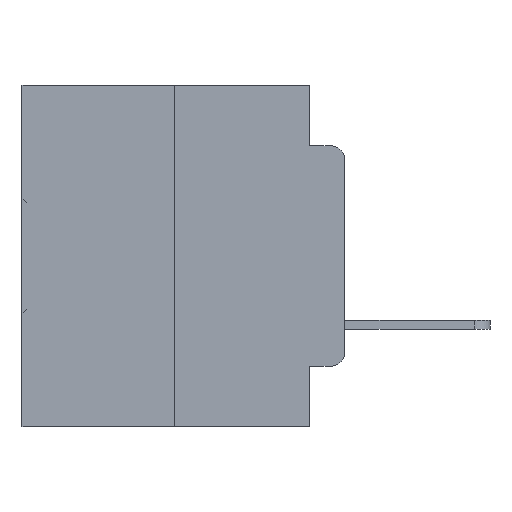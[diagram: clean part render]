
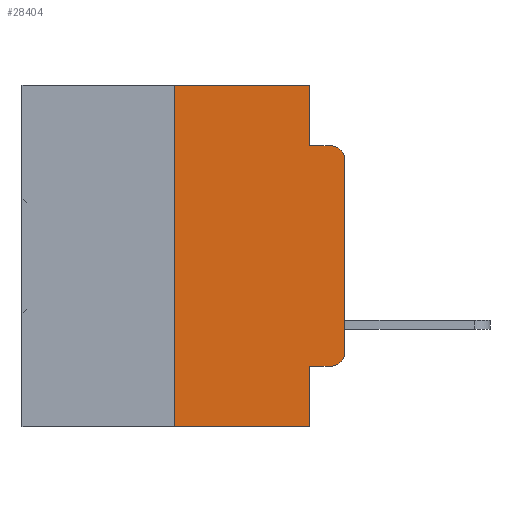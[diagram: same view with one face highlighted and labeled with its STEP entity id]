
A CAD part, left-side view. The second image highlights one B-rep face of the part: STEP entity #28404.
In plain terms, the highlighted planar face has unit normal (-1, 0, 0).
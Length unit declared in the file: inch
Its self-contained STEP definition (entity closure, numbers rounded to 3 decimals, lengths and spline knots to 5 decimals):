
#94 = AXIS2_PLACEMENT_3D ( 'NONE', #10459, #28634, #13174 ) ;
#438 = LINE ( 'NONE', #4301, #14410 ) ;
#496 = CARTESIAN_POINT ( 'NONE',  ( 0., 0.051, 0. ) ) ;
#543 = LINE ( 'NONE', #33688, #28197 ) ;
#1624 = LINE ( 'NONE', #32157, #21797 ) ;
#1971 = VERTEX_POINT ( 'NONE', #26791 ) ;
#1994 = ORIENTED_EDGE ( 'NONE', *, *, #27811, .F. ) ;
#2024 = PLANE ( 'NONE',  #94 ) ;
#2053 = DIRECTION ( 'NONE',  ( -1., 0., 0. ) ) ;
#2363 = CARTESIAN_POINT ( 'NONE',  ( 0., 0., -0.1085 ) ) ;
#2438 = ORIENTED_EDGE ( 'NONE', *, *, #27023, .T. ) ;
#2786 = CARTESIAN_POINT ( 'NONE',  ( 0., 0.051, -0.5 ) ) ;
#3160 = EDGE_CURVE ( 'NONE', #33085, #18501, #29406, .T. ) ;
#3430 = DIRECTION ( 'NONE',  ( 0., 0., -1. ) ) ;
#3514 = VERTEX_POINT ( 'NONE', #20833 ) ;
#4301 = CARTESIAN_POINT ( 'NONE',  ( 0., 0.051, -0.0885 ) ) ;
#4998 = EDGE_CURVE ( 'NONE', #33827, #24854, #438, .T. ) ;
#5915 = ORIENTED_EDGE ( 'NONE', *, *, #30464, .F. ) ;
#6260 = DIRECTION ( 'NONE',  ( 0., -1., 0. ) ) ;
#6485 = VECTOR ( 'NONE', #3430, 39.37008 ) ;
#7078 = DIRECTION ( 'NONE',  ( 0., -1., 0. ) ) ;
#7721 = AXIS2_PLACEMENT_3D ( 'NONE', #18683, #2053, #21248 ) ;
#10459 = CARTESIAN_POINT ( 'NONE',  ( 0., 0.473, 0. ) ) ;
#10749 = CIRCLE ( 'NONE', #7721, 0.02 ) ;
#10888 = DIRECTION ( 'NONE',  ( 0., -1., 0. ) ) ;
#11348 = CARTESIAN_POINT ( 'NONE',  ( 0., 0.051, -0.4115 ) ) ;
#11583 = ORIENTED_EDGE ( 'NONE', *, *, #4998, .F. ) ;
#11832 = CARTESIAN_POINT ( 'NONE',  ( 0., 0., -0.3915 ) ) ;
#12971 = LINE ( 'NONE', #496, #6485 ) ;
#13174 = DIRECTION ( 'NONE',  ( 0., 0., -1. ) ) ;
#13966 = EDGE_CURVE ( 'NONE', #29970, #24553, #543, .T. ) ;
#14148 = CARTESIAN_POINT ( 'NONE',  ( 0., 0.051, 0. ) ) ;
#14410 = VECTOR ( 'NONE', #7078, 39.37008 ) ;
#14554 = DIRECTION ( 'NONE',  ( -1., 0., 0. ) ) ;
#14745 = CARTESIAN_POINT ( 'NONE',  ( 0., 0.051, -0.0885 ) ) ;
#14992 = ORIENTED_EDGE ( 'NONE', *, *, #19322, .F. ) ;
#15796 = EDGE_CURVE ( 'NONE', #29505, #33085, #10749, .T. ) ;
#17017 = CARTESIAN_POINT ( 'NONE',  ( 0., 0.02, -0.4115 ) ) ;
#17399 = LINE ( 'NONE', #29879, #29911 ) ;
#18284 = VECTOR ( 'NONE', #30911, 39.37008 ) ;
#18358 = EDGE_CURVE ( 'NONE', #1971, #3514, #31389, .T. ) ;
#18482 = CARTESIAN_POINT ( 'NONE',  ( 0., 0.25, -0.5 ) ) ;
#18501 = VERTEX_POINT ( 'NONE', #2363 ) ;
#18683 = CARTESIAN_POINT ( 'NONE',  ( 0., 0.02, -0.3915 ) ) ;
#19322 = EDGE_CURVE ( 'NONE', #29970, #1971, #17399, .T. ) ;
#20078 = DIRECTION ( 'NONE',  ( 0., 0., 1. ) ) ;
#20529 = ORIENTED_EDGE ( 'NONE', *, *, #18358, .F. ) ;
#20833 = CARTESIAN_POINT ( 'NONE',  ( 0., 0.051, 0. ) ) ;
#21248 = DIRECTION ( 'NONE',  ( 0., 0., -1. ) ) ;
#21535 = VERTEX_POINT ( 'NONE', #11348 ) ;
#21797 = VECTOR ( 'NONE', #6260, 39.37008 ) ;
#22100 = ORIENTED_EDGE ( 'NONE', *, *, #13966, .T. ) ;
#22241 = DIRECTION ( 'NONE',  ( 0., 0., -1. ) ) ;
#22767 = FACE_OUTER_BOUND ( 'NONE', #25548, .T. ) ;
#23261 = ORIENTED_EDGE ( 'NONE', *, *, #3160, .T. ) ;
#23648 = ORIENTED_EDGE ( 'NONE', *, *, #31011, .T. ) ;
#23689 = VECTOR ( 'NONE', #33490, 39.37008 ) ;
#23912 = CARTESIAN_POINT ( 'NONE',  ( 0., 0., 0. ) ) ;
#24553 = VERTEX_POINT ( 'NONE', #2786 ) ;
#24672 = AXIS2_PLACEMENT_3D ( 'NONE', #29859, #14554, #32242 ) ;
#24854 = VERTEX_POINT ( 'NONE', #26090 ) ;
#25548 = EDGE_LOOP ( 'NONE', ( #23261, #2438, #11583, #5915, #20529, #14992, #22100, #1994, #23648, #30124 ) ) ;
#26090 = CARTESIAN_POINT ( 'NONE',  ( 0., 0.02, -0.0885 ) ) ;
#26791 = CARTESIAN_POINT ( 'NONE',  ( 0., 0.25, 0. ) ) ;
#27023 = EDGE_CURVE ( 'NONE', #18501, #24854, #30070, .T. ) ;
#27790 = LINE ( 'NONE', #14148, #33373 ) ;
#27811 = EDGE_CURVE ( 'NONE', #21535, #24553, #27790, .T. ) ;
#28197 = VECTOR ( 'NONE', #10888, 39.37008 ) ;
#28404 = ADVANCED_FACE ( 'NONE', ( #22767 ), #2024, .F. ) ;
#28500 = CARTESIAN_POINT ( 'NONE',  ( 0., 0.473, 0. ) ) ;
#28634 = DIRECTION ( 'NONE',  ( 1., 0., 0. ) ) ;
#29406 = LINE ( 'NONE', #23912, #23689 ) ;
#29505 = VERTEX_POINT ( 'NONE', #17017 ) ;
#29859 = CARTESIAN_POINT ( 'NONE',  ( 0., 0.02, -0.1085 ) ) ;
#29879 = CARTESIAN_POINT ( 'NONE',  ( 0., 0.25, 0. ) ) ;
#29911 = VECTOR ( 'NONE', #20078, 39.37008 ) ;
#29970 = VERTEX_POINT ( 'NONE', #18482 ) ;
#30070 = CIRCLE ( 'NONE', #24672, 0.02 ) ;
#30124 = ORIENTED_EDGE ( 'NONE', *, *, #15796, .T. ) ;
#30464 = EDGE_CURVE ( 'NONE', #3514, #33827, #12971, .T. ) ;
#30911 = DIRECTION ( 'NONE',  ( 0., -1., 0. ) ) ;
#31011 = EDGE_CURVE ( 'NONE', #21535, #29505, #1624, .T. ) ;
#31389 = LINE ( 'NONE', #28500, #18284 ) ;
#32157 = CARTESIAN_POINT ( 'NONE',  ( 0., 0.051, -0.4115 ) ) ;
#32242 = DIRECTION ( 'NONE',  ( 0., 0., -1. ) ) ;
#33085 = VERTEX_POINT ( 'NONE', #11832 ) ;
#33373 = VECTOR ( 'NONE', #22241, 39.37008 ) ;
#33490 = DIRECTION ( 'NONE',  ( 0., 0., 1. ) ) ;
#33688 = CARTESIAN_POINT ( 'NONE',  ( 0., 0.473, -0.5 ) ) ;
#33827 = VERTEX_POINT ( 'NONE', #14745 ) ;
